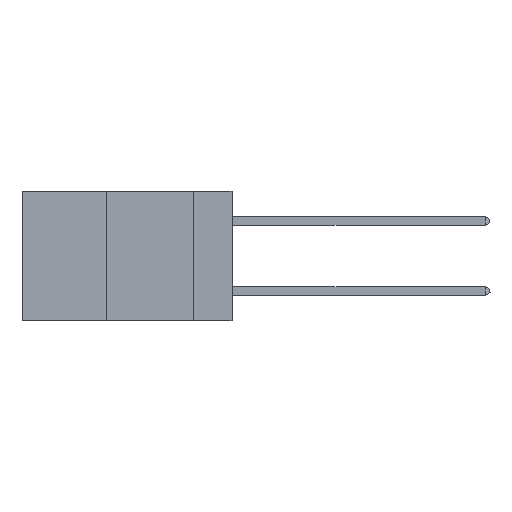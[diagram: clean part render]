
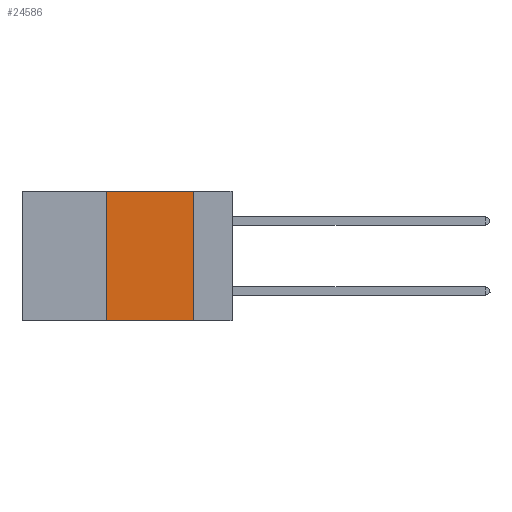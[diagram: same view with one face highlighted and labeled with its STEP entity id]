
A CAD part, left-side view. The second image highlights one B-rep face of the part: STEP entity #24586.
In plain terms, the highlighted planar face has unit normal (-1, 0, 0).
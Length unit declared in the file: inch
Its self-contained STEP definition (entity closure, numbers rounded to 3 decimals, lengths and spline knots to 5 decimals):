
#652 = EDGE_CURVE ( 'NONE', #28075, #40315, #31523, .T. ) ;
#789 = DIRECTION ( 'NONE',  ( 1., 0., 0. ) ) ;
#1649 = LINE ( 'NONE', #30207, #36254 ) ;
#6140 = CARTESIAN_POINT ( 'NONE',  ( 0., 0.6, 0. ) ) ;
#8689 = DIRECTION ( 'NONE',  ( 0., 0., -1. ) ) ;
#9325 = DIRECTION ( 'NONE',  ( 0., -1., 0. ) ) ;
#10076 = EDGE_CURVE ( 'NONE', #40315, #41394, #30177, .T. ) ;
#11072 = CARTESIAN_POINT ( 'NONE',  ( 0., 0.36, 0. ) ) ;
#12523 = CARTESIAN_POINT ( 'NONE',  ( 0., 0.6, -0.37 ) ) ;
#13396 = VECTOR ( 'NONE', #8689, 39.37008 ) ;
#13776 = DIRECTION ( 'NONE',  ( 0., 0., 1. ) ) ;
#15260 = AXIS2_PLACEMENT_3D ( 'NONE', #27283, #789, #34457 ) ;
#15713 = CARTESIAN_POINT ( 'NONE',  ( 0., 0.11, -0.37 ) ) ;
#17065 = EDGE_LOOP ( 'NONE', ( #23459, #41860, #24518, #21904 ) ) ;
#20137 = VECTOR ( 'NONE', #42957, 39.37008 ) ;
#21904 = ORIENTED_EDGE ( 'NONE', *, *, #22154, .T. ) ;
#22154 = EDGE_CURVE ( 'NONE', #31762, #41394, #24785, .T. ) ;
#23459 = ORIENTED_EDGE ( 'NONE', *, *, #10076, .F. ) ;
#24518 = ORIENTED_EDGE ( 'NONE', *, *, #29673, .F. ) ;
#24586 = ADVANCED_FACE ( 'NONE', ( #38196 ), #30960, .F. ) ;
#24607 = CARTESIAN_POINT ( 'NONE',  ( 0., 0.36, -0.37 ) ) ;
#24785 = LINE ( 'NONE', #12523, #20137 ) ;
#25096 = CARTESIAN_POINT ( 'NONE',  ( 0., 0.11, 0. ) ) ;
#27283 = CARTESIAN_POINT ( 'NONE',  ( 0., 0.6, 0. ) ) ;
#27917 = CARTESIAN_POINT ( 'NONE',  ( 0., 0.11, 0. ) ) ;
#28075 = VERTEX_POINT ( 'NONE', #11072 ) ;
#29673 = EDGE_CURVE ( 'NONE', #31762, #28075, #1649, .T. ) ;
#30177 = LINE ( 'NONE', #25096, #13396 ) ;
#30207 = CARTESIAN_POINT ( 'NONE',  ( 0., 0.36, 0. ) ) ;
#30960 = PLANE ( 'NONE',  #15260 ) ;
#31523 = LINE ( 'NONE', #6140, #36241 ) ;
#31762 = VERTEX_POINT ( 'NONE', #24607 ) ;
#34457 = DIRECTION ( 'NONE',  ( 0., 0., -1. ) ) ;
#36241 = VECTOR ( 'NONE', #9325, 39.37008 ) ;
#36254 = VECTOR ( 'NONE', #13776, 39.37008 ) ;
#38196 = FACE_OUTER_BOUND ( 'NONE', #17065, .T. ) ;
#40315 = VERTEX_POINT ( 'NONE', #27917 ) ;
#41394 = VERTEX_POINT ( 'NONE', #15713 ) ;
#41860 = ORIENTED_EDGE ( 'NONE', *, *, #652, .F. ) ;
#42957 = DIRECTION ( 'NONE',  ( 0., -1., 0. ) ) ;
